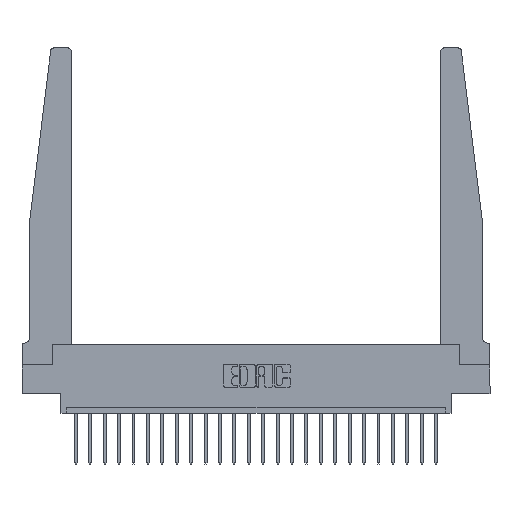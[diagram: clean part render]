
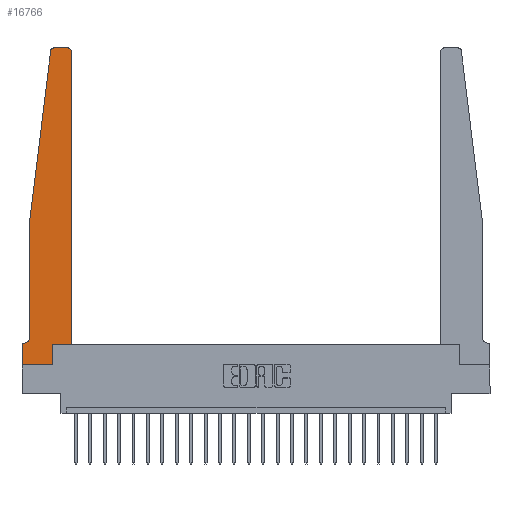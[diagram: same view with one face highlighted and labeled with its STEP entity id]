
A CAD part, top view. The second image highlights one B-rep face of the part: STEP entity #16766.
In plain terms, the highlighted planar face has unit normal (0, 0, 1).
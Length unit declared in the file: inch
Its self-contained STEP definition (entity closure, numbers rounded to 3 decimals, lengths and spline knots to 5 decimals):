
#331 = DIRECTION ( 'NONE',  ( 1., 0., 0. ) ) ;
#389 = EDGE_CURVE ( 'NONE', #16707, #21837, #2437, .T. ) ;
#666 = LINE ( 'NONE', #10233, #18616 ) ;
#806 = DIRECTION ( 'NONE',  ( 0., 0., 1. ) ) ;
#871 = CARTESIAN_POINT ( 'NONE',  ( 0.395, 2.75, 0.37 ) ) ;
#955 = ORIENTED_EDGE ( 'NONE', *, *, #15144, .T. ) ;
#999 = ORIENTED_EDGE ( 'NONE', *, *, #2393, .T. ) ;
#1024 = VECTOR ( 'NONE', #15508, 39.37008 ) ;
#1193 = CARTESIAN_POINT ( 'NONE',  ( 0.25, 2.75, 0.37 ) ) ;
#1209 = EDGE_CURVE ( 'NONE', #16729, #11288, #5803, .T. ) ;
#1374 = CARTESIAN_POINT ( 'NONE',  ( 0.2605, 0.18, 0.37 ) ) ;
#1602 = DIRECTION ( 'NONE',  ( -1., 0., 0. ) ) ;
#1718 = DIRECTION ( 'NONE',  ( 0., 1., 0. ) ) ;
#1797 = CARTESIAN_POINT ( 'NONE',  ( 0.425, 2.72, 0.37 ) ) ;
#2145 = ORIENTED_EDGE ( 'NONE', *, *, #389, .T. ) ;
#2227 = EDGE_CURVE ( 'NONE', #22138, #15868, #11372, .T. ) ;
#2393 = EDGE_CURVE ( 'NONE', #3549, #5910, #9952, .T. ) ;
#2437 = LINE ( 'NONE', #17602, #5000 ) ;
#2510 = EDGE_CURVE ( 'NONE', #21837, #16729, #7685, .T. ) ;
#2668 = ORIENTED_EDGE ( 'NONE', *, *, #12287, .T. ) ;
#2913 = VECTOR ( 'NONE', #5245, 39.37008 ) ;
#2933 = ORIENTED_EDGE ( 'NONE', *, *, #19330, .T. ) ;
#3102 = DIRECTION ( 'NONE',  ( 0., 1., 0. ) ) ;
#3188 = DIRECTION ( 'NONE',  ( -1., 0., 0. ) ) ;
#3375 = VERTEX_POINT ( 'NONE', #20871 ) ;
#3549 = VERTEX_POINT ( 'NONE', #22817 ) ;
#3662 = CARTESIAN_POINT ( 'NONE',  ( 0.065, 0.2375, 0.37 ) ) ;
#4181 = PLANE ( 'NONE',  #10021 ) ;
#4278 = LINE ( 'NONE', #22377, #11845 ) ;
#4603 = DIRECTION ( 'NONE',  ( 0., 0., 1. ) ) ;
#5000 = VECTOR ( 'NONE', #1602, 39.37008 ) ;
#5090 = CARTESIAN_POINT ( 'NONE',  ( 0.015, 0.2375, 0.37 ) ) ;
#5228 = DIRECTION ( 'NONE',  ( 1., 0., 0. ) ) ;
#5245 = DIRECTION ( 'NONE',  ( 0., -1., 0. ) ) ;
#5583 = VECTOR ( 'NONE', #3102, 39.37008 ) ;
#5803 = LINE ( 'NONE', #8221, #1024 ) ;
#5910 = VERTEX_POINT ( 'NONE', #12836 ) ;
#6533 = CARTESIAN_POINT ( 'NONE',  ( 0., 0.1875, 0.37 ) ) ;
#6784 = VERTEX_POINT ( 'NONE', #3662 ) ;
#6840 = VERTEX_POINT ( 'NONE', #13005 ) ;
#6916 = CARTESIAN_POINT ( 'NONE',  ( 0.425, 0.18, 0.37 ) ) ;
#7685 = LINE ( 'NONE', #15958, #2913 ) ;
#8221 = CARTESIAN_POINT ( 'NONE',  ( 0., 0., 0.37 ) ) ;
#8296 = CARTESIAN_POINT ( 'NONE',  ( 0.27653, 2.72, 0.37 ) ) ;
#8317 = CARTESIAN_POINT ( 'NONE',  ( 0.065, 1.25, 0.37 ) ) ;
#9952 = CIRCLE ( 'NONE', #17625, 0.03 ) ;
#10021 = AXIS2_PLACEMENT_3D ( 'NONE', #22166, #20242, #331 ) ;
#10233 = CARTESIAN_POINT ( 'NONE',  ( 0.425, 0.18, 0.37 ) ) ;
#10696 = LINE ( 'NONE', #1193, #22423 ) ;
#11288 = VERTEX_POINT ( 'NONE', #12561 ) ;
#11347 = VERTEX_POINT ( 'NONE', #18117 ) ;
#11372 = CIRCLE ( 'NONE', #21960, 0.03 ) ;
#11835 = DIRECTION ( 'NONE',  ( 1., 0., 0. ) ) ;
#11845 = VECTOR ( 'NONE', #20673, 39.37008 ) ;
#11890 = EDGE_CURVE ( 'NONE', #11347, #6840, #20976, .T. ) ;
#12287 = EDGE_CURVE ( 'NONE', #11288, #11347, #18451, .T. ) ;
#12561 = CARTESIAN_POINT ( 'NONE',  ( 0.2605, 0., 0.37 ) ) ;
#12836 = CARTESIAN_POINT ( 'NONE',  ( 0.24675, 2.72367, 0.37 ) ) ;
#13005 = CARTESIAN_POINT ( 'NONE',  ( 0.425, 0.18, 0.37 ) ) ;
#13173 = LINE ( 'NONE', #8317, #19046 ) ;
#13875 = DIRECTION ( 'NONE',  ( 0., 0., -1. ) ) ;
#14690 = EDGE_CURVE ( 'NONE', #5910, #3375, #4278, .T. ) ;
#15117 = FACE_OUTER_BOUND ( 'NONE', #16962, .T. ) ;
#15144 = EDGE_CURVE ( 'NONE', #15868, #3549, #10696, .T. ) ;
#15508 = DIRECTION ( 'NONE',  ( 1., 0., 0. ) ) ;
#15868 = VERTEX_POINT ( 'NONE', #871 ) ;
#15900 = DIRECTION ( 'NONE',  ( 0., -1., 0. ) ) ;
#15958 = CARTESIAN_POINT ( 'NONE',  ( 0., 0., 0.37 ) ) ;
#16341 = CARTESIAN_POINT ( 'NONE',  ( 0., 0., 0.37 ) ) ;
#16349 = EDGE_CURVE ( 'NONE', #3375, #6784, #13173, .T. ) ;
#16416 = CARTESIAN_POINT ( 'NONE',  ( 0.015, 0.1875, 0.37 ) ) ;
#16611 = ORIENTED_EDGE ( 'NONE', *, *, #14690, .T. ) ;
#16707 = VERTEX_POINT ( 'NONE', #16416 ) ;
#16729 = VERTEX_POINT ( 'NONE', #16341 ) ;
#16766 = ADVANCED_FACE ( 'NONE', ( #15117 ), #4181, .T. ) ;
#16962 = EDGE_LOOP ( 'NONE', ( #955, #999, #16611, #22573, #19487, #2145, #18866, #22851, #2668, #19606, #2933, #22692 ) ) ;
#17430 = DIRECTION ( 'NONE',  ( 1., 0., 0. ) ) ;
#17602 = CARTESIAN_POINT ( 'NONE',  ( 0.065, 0.1875, 0.37 ) ) ;
#17625 = AXIS2_PLACEMENT_3D ( 'NONE', #8296, #4603, #11835 ) ;
#18117 = CARTESIAN_POINT ( 'NONE',  ( 0.2605, 0.18, 0.37 ) ) ;
#18451 = LINE ( 'NONE', #1374, #5583 ) ;
#18616 = VECTOR ( 'NONE', #1718, 39.37008 ) ;
#18866 = ORIENTED_EDGE ( 'NONE', *, *, #2510, .T. ) ;
#19046 = VECTOR ( 'NONE', #15900, 39.37008 ) ;
#19153 = DIRECTION ( 'NONE',  ( -1., 0., 0. ) ) ;
#19330 = EDGE_CURVE ( 'NONE', #6840, #22138, #666, .T. ) ;
#19487 = ORIENTED_EDGE ( 'NONE', *, *, #22948, .T. ) ;
#19606 = ORIENTED_EDGE ( 'NONE', *, *, #11890, .T. ) ;
#20242 = DIRECTION ( 'NONE',  ( 0., 0., 1. ) ) ;
#20673 = DIRECTION ( 'NONE',  ( -0.122, -0.992, 0. ) ) ;
#20871 = CARTESIAN_POINT ( 'NONE',  ( 0.065, 1.25, 0.37 ) ) ;
#20976 = LINE ( 'NONE', #6916, #22648 ) ;
#21638 = AXIS2_PLACEMENT_3D ( 'NONE', #5090, #13875, #3188 ) ;
#21837 = VERTEX_POINT ( 'NONE', #6533 ) ;
#21960 = AXIS2_PLACEMENT_3D ( 'NONE', #22411, #806, #17430 ) ;
#22138 = VERTEX_POINT ( 'NONE', #1797 ) ;
#22166 = CARTESIAN_POINT ( 'NONE',  ( 0., 0.1875, 0.37 ) ) ;
#22377 = CARTESIAN_POINT ( 'NONE',  ( 0.065, 1.25, 0.37 ) ) ;
#22411 = CARTESIAN_POINT ( 'NONE',  ( 0.395, 2.72, 0.37 ) ) ;
#22423 = VECTOR ( 'NONE', #19153, 39.37008 ) ;
#22531 = CIRCLE ( 'NONE', #21638, 0.05 ) ;
#22573 = ORIENTED_EDGE ( 'NONE', *, *, #16349, .T. ) ;
#22648 = VECTOR ( 'NONE', #5228, 39.37008 ) ;
#22692 = ORIENTED_EDGE ( 'NONE', *, *, #2227, .T. ) ;
#22817 = CARTESIAN_POINT ( 'NONE',  ( 0.27653, 2.75, 0.37 ) ) ;
#22851 = ORIENTED_EDGE ( 'NONE', *, *, #1209, .T. ) ;
#22948 = EDGE_CURVE ( 'NONE', #6784, #16707, #22531, .T. ) ;
